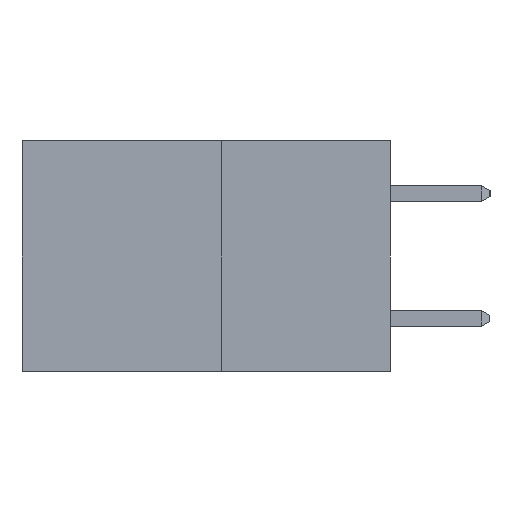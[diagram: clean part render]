
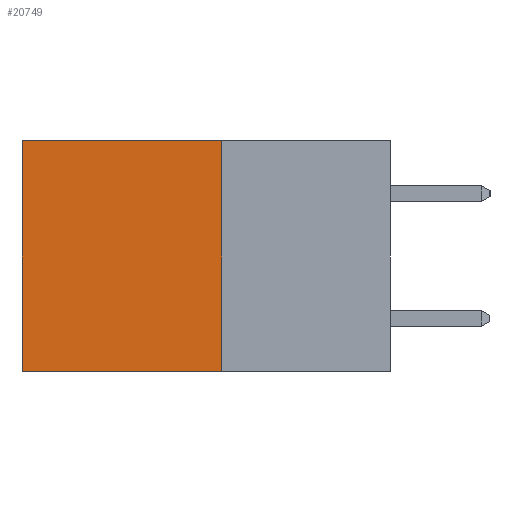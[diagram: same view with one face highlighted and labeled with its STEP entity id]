
A CAD part, left-side view. The second image highlights one B-rep face of the part: STEP entity #20749.
In plain terms, the highlighted planar face has unit normal (-1, 0, 0).
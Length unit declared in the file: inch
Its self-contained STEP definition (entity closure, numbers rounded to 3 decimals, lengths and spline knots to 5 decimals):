
#376 = PLANE ( 'NONE',  #3357 ) ;
#2169 = DIRECTION ( 'NONE',  ( 1., 0., 0. ) ) ;
#2441 = VERTEX_POINT ( 'NONE', #18992 ) ;
#2607 = VECTOR ( 'NONE', #11085, 39.37008 ) ;
#2678 = ORIENTED_EDGE ( 'NONE', *, *, #21144, .T. ) ;
#2719 = ORIENTED_EDGE ( 'NONE', *, *, #8872, .F. ) ;
#2887 = ORIENTED_EDGE ( 'NONE', *, *, #11664, .F. ) ;
#2911 = ORIENTED_EDGE ( 'NONE', *, *, #15223, .T. ) ;
#2958 = VERTEX_POINT ( 'NONE', #16306 ) ;
#3237 = VERTEX_POINT ( 'NONE', #4428 ) ;
#3357 = AXIS2_PLACEMENT_3D ( 'NONE', #17766, #2169, #14366 ) ;
#4428 = CARTESIAN_POINT ( 'NONE',  ( 0.277, 0.59, -0.37 ) ) ;
#6663 = VECTOR ( 'NONE', #15429, 39.37008 ) ;
#8872 = EDGE_CURVE ( 'NONE', #2441, #9613, #16508, .T. ) ;
#9273 = CARTESIAN_POINT ( 'NONE',  ( 0.277, 0.27, -0.37 ) ) ;
#9319 = CARTESIAN_POINT ( 'NONE',  ( 0.277, 0.27, -0.37 ) ) ;
#9608 = VECTOR ( 'NONE', #11943, 39.37008 ) ;
#9613 = VERTEX_POINT ( 'NONE', #12681 ) ;
#11085 = DIRECTION ( 'NONE',  ( 0., 0., -1. ) ) ;
#11664 = EDGE_CURVE ( 'NONE', #9613, #3237, #21716, .T. ) ;
#11943 = DIRECTION ( 'NONE',  ( 0., 0., -1. ) ) ;
#12681 = CARTESIAN_POINT ( 'NONE',  ( 0.277, 0.27, -0.37 ) ) ;
#13508 = EDGE_LOOP ( 'NONE', ( #2911, #2887, #2719, #2678 ) ) ;
#13624 = LINE ( 'NONE', #22230, #9608 ) ;
#13652 = VECTOR ( 'NONE', #19803, 39.37008 ) ;
#13658 = CARTESIAN_POINT ( 'NONE',  ( 0.277, 0.27, 0. ) ) ;
#14366 = DIRECTION ( 'NONE',  ( 0., 0., -1. ) ) ;
#14790 = FACE_OUTER_BOUND ( 'NONE', #13508, .T. ) ;
#15223 = EDGE_CURVE ( 'NONE', #2958, #3237, #13624, .T. ) ;
#15429 = DIRECTION ( 'NONE',  ( 0., 1., 0. ) ) ;
#15855 = LINE ( 'NONE', #13658, #6663 ) ;
#16306 = CARTESIAN_POINT ( 'NONE',  ( 0.277, 0.59, 0. ) ) ;
#16508 = LINE ( 'NONE', #9273, #2607 ) ;
#17766 = CARTESIAN_POINT ( 'NONE',  ( 0.277, 0.27, -0.37 ) ) ;
#18992 = CARTESIAN_POINT ( 'NONE',  ( 0.277, 0.27, 0. ) ) ;
#19803 = DIRECTION ( 'NONE',  ( 0., 1., 0. ) ) ;
#20749 = ADVANCED_FACE ( 'NONE', ( #14790 ), #376, .F. ) ;
#21144 = EDGE_CURVE ( 'NONE', #2441, #2958, #15855, .T. ) ;
#21716 = LINE ( 'NONE', #9319, #13652 ) ;
#22230 = CARTESIAN_POINT ( 'NONE',  ( 0.277, 0.59, -0.37 ) ) ;
